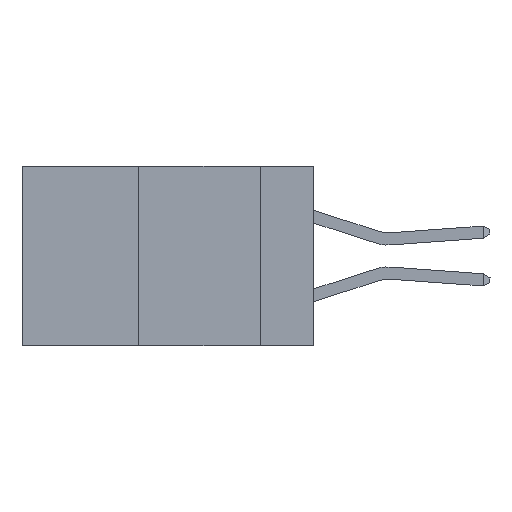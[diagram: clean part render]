
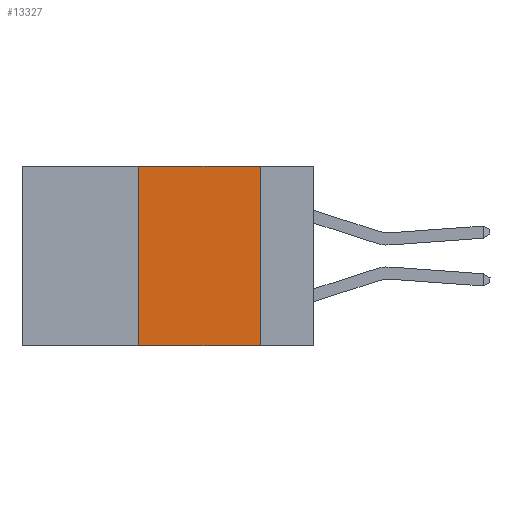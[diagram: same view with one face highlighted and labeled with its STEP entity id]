
A CAD part, left-side view. The second image highlights one B-rep face of the part: STEP entity #13327.
In plain terms, the highlighted planar face has unit normal (-1, 0, 0).
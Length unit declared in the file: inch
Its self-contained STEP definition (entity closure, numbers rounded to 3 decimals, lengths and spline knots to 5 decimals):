
#543 = DIRECTION ( 'NONE',  ( 0., 0., -1. ) ) ;
#1029 = VECTOR ( 'NONE', #543, 39.37008 ) ;
#1618 = ORIENTED_EDGE ( 'NONE', *, *, #7893, .F. ) ;
#1683 = CARTESIAN_POINT ( 'NONE',  ( 0., 0.11, -0.37 ) ) ;
#1806 = ORIENTED_EDGE ( 'NONE', *, *, #20605, .T. ) ;
#3124 = LINE ( 'NONE', #30448, #1029 ) ;
#3520 = CARTESIAN_POINT ( 'NONE',  ( 0., 0.11, 0. ) ) ;
#3977 = EDGE_CURVE ( 'NONE', #8040, #31961, #3124, .T. ) ;
#5203 = FACE_OUTER_BOUND ( 'NONE', #32010, .T. ) ;
#5363 = CARTESIAN_POINT ( 'NONE',  ( 0., 0.6, -0.37 ) ) ;
#7893 = EDGE_CURVE ( 'NONE', #17817, #8040, #15942, .T. ) ;
#8040 = VERTEX_POINT ( 'NONE', #3520 ) ;
#8068 = VECTOR ( 'NONE', #29752, 39.37008 ) ;
#13327 = ADVANCED_FACE ( 'NONE', ( #5203 ), #18223, .F. ) ;
#14758 = DIRECTION ( 'NONE',  ( 0., -1., 0. ) ) ;
#15025 = LINE ( 'NONE', #5363, #25507 ) ;
#15942 = LINE ( 'NONE', #23175, #8068 ) ;
#16400 = AXIS2_PLACEMENT_3D ( 'NONE', #34652, #41725, #21565 ) ;
#17817 = VERTEX_POINT ( 'NONE', #28672 ) ;
#18223 = PLANE ( 'NONE',  #16400 ) ;
#20605 = EDGE_CURVE ( 'NONE', #36259, #31961, #15025, .T. ) ;
#21565 = DIRECTION ( 'NONE',  ( 0., 0., -1. ) ) ;
#23175 = CARTESIAN_POINT ( 'NONE',  ( 0., 0.6, 0. ) ) ;
#25507 = VECTOR ( 'NONE', #14758, 39.37008 ) ;
#28413 = ORIENTED_EDGE ( 'NONE', *, *, #3977, .F. ) ;
#28672 = CARTESIAN_POINT ( 'NONE',  ( 0., 0.36, 0. ) ) ;
#29122 = ORIENTED_EDGE ( 'NONE', *, *, #29156, .F. ) ;
#29156 = EDGE_CURVE ( 'NONE', #36259, #17817, #43157, .T. ) ;
#29473 = VECTOR ( 'NONE', #39510, 39.37008 ) ;
#29752 = DIRECTION ( 'NONE',  ( 0., -1., 0. ) ) ;
#30448 = CARTESIAN_POINT ( 'NONE',  ( 0., 0.11, 0. ) ) ;
#31961 = VERTEX_POINT ( 'NONE', #1683 ) ;
#32010 = EDGE_LOOP ( 'NONE', ( #28413, #1618, #29122, #1806 ) ) ;
#32390 = CARTESIAN_POINT ( 'NONE',  ( 0., 0.36, 0. ) ) ;
#34652 = CARTESIAN_POINT ( 'NONE',  ( 0., 0.6, 0. ) ) ;
#36259 = VERTEX_POINT ( 'NONE', #42560 ) ;
#39510 = DIRECTION ( 'NONE',  ( 0., 0., 1. ) ) ;
#41725 = DIRECTION ( 'NONE',  ( 1., 0., 0. ) ) ;
#42560 = CARTESIAN_POINT ( 'NONE',  ( 0., 0.36, -0.37 ) ) ;
#43157 = LINE ( 'NONE', #32390, #29473 ) ;
